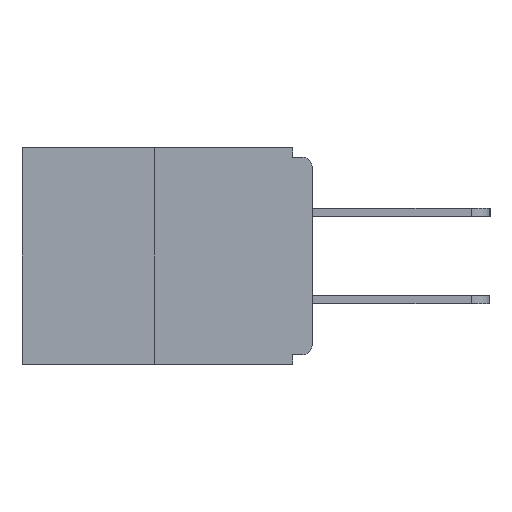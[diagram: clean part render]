
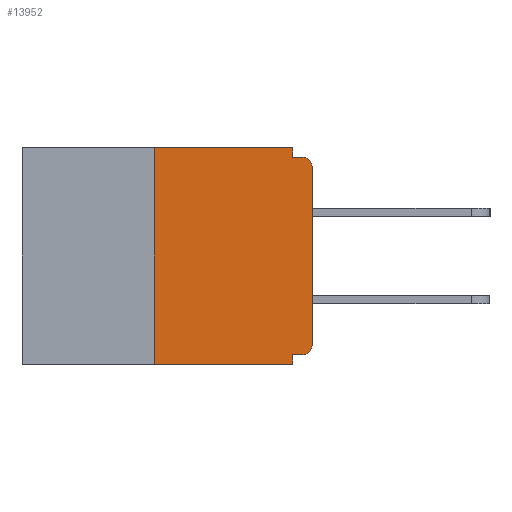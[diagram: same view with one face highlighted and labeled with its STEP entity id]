
A CAD part, left-side view. The second image highlights one B-rep face of the part: STEP entity #13952.
In plain terms, the highlighted planar face has unit normal (-1, 0, 0).
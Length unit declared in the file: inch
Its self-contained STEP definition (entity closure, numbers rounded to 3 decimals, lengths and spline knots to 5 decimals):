
#26 = CARTESIAN_POINT ( 'NONE',  ( 0., 0.46, -0.343 ) ) ;
#234 = EDGE_CURVE ( 'NONE', #9719, #2152, #12097, .T. ) ;
#257 = EDGE_CURVE ( 'NONE', #15197, #10147, #7958, .T. ) ;
#394 = CARTESIAN_POINT ( 'NONE',  ( 0., 0.25, 0. ) ) ;
#499 = DIRECTION ( 'NONE',  ( -1., 0., 0. ) ) ;
#821 = CARTESIAN_POINT ( 'NONE',  ( 0., 0.015, -0.015 ) ) ;
#1086 = CARTESIAN_POINT ( 'NONE',  ( 0., 0.25, -0.343 ) ) ;
#1186 = DIRECTION ( 'NONE',  ( 0., 0., 1. ) ) ;
#1249 = VERTEX_POINT ( 'NONE', #8671 ) ;
#1519 = CIRCLE ( 'NONE', #7314, 0.015 ) ;
#1604 = LINE ( 'NONE', #6261, #15446 ) ;
#1850 = PLANE ( 'NONE',  #8374 ) ;
#2152 = VERTEX_POINT ( 'NONE', #6568 ) ;
#2819 = VECTOR ( 'NONE', #16020, 39.37008 ) ;
#3229 = DIRECTION ( 'NONE',  ( 0., -1., 0. ) ) ;
#3533 = ORIENTED_EDGE ( 'NONE', *, *, #234, .F. ) ;
#3569 = EDGE_CURVE ( 'NONE', #5611, #10739, #1604, .T. ) ;
#3644 = VECTOR ( 'NONE', #16268, 39.37008 ) ;
#3814 = VERTEX_POINT ( 'NONE', #821 ) ;
#4016 = CARTESIAN_POINT ( 'NONE',  ( 0., 0., -0.328 ) ) ;
#4102 = ORIENTED_EDGE ( 'NONE', *, *, #6566, .T. ) ;
#4181 = EDGE_CURVE ( 'NONE', #9719, #10739, #6935, .T. ) ;
#4430 = DIRECTION ( 'NONE',  ( 0., 0., -1. ) ) ;
#4498 = LINE ( 'NONE', #4016, #2819 ) ;
#4699 = LINE ( 'NONE', #8275, #9035 ) ;
#4856 = CIRCLE ( 'NONE', #13035, 0.015 ) ;
#5150 = EDGE_CURVE ( 'NONE', #2152, #15197, #4699, .T. ) ;
#5329 = VECTOR ( 'NONE', #13283, 39.37008 ) ;
#5611 = VERTEX_POINT ( 'NONE', #9709 ) ;
#5800 = ORIENTED_EDGE ( 'NONE', *, *, #257, .F. ) ;
#6261 = CARTESIAN_POINT ( 'NONE',  ( 0., 0.031, -0.343 ) ) ;
#6269 = DIRECTION ( 'NONE',  ( 0., 0., -1. ) ) ;
#6470 = EDGE_LOOP ( 'NONE', ( #12207, #3533, #7846, #15551, #7642, #4102, #16042, #11054, #15247, #5800 ) ) ;
#6566 = EDGE_CURVE ( 'NONE', #14344, #16551, #4856, .T. ) ;
#6568 = CARTESIAN_POINT ( 'NONE',  ( 0., 0.25, 0. ) ) ;
#6770 = CARTESIAN_POINT ( 'NONE',  ( 0., 0.015, -0.328 ) ) ;
#6935 = LINE ( 'NONE', #26, #5329 ) ;
#6994 = DIRECTION ( 'NONE',  ( 0., 0., 1. ) ) ;
#7049 = CARTESIAN_POINT ( 'NONE',  ( 0., 0.031, 0. ) ) ;
#7126 = CARTESIAN_POINT ( 'NONE',  ( 0., 0.031, -0.015 ) ) ;
#7143 = DIRECTION ( 'NONE',  ( 0., 0., -1. ) ) ;
#7314 = AXIS2_PLACEMENT_3D ( 'NONE', #8338, #499, #4430 ) ;
#7642 = ORIENTED_EDGE ( 'NONE', *, *, #15091, .F. ) ;
#7813 = CARTESIAN_POINT ( 'NONE',  ( 0., 0., -0.313 ) ) ;
#7846 = ORIENTED_EDGE ( 'NONE', *, *, #4181, .T. ) ;
#7951 = FACE_OUTER_BOUND ( 'NONE', #6470, .T. ) ;
#7958 = LINE ( 'NONE', #7049, #3644 ) ;
#8275 = CARTESIAN_POINT ( 'NONE',  ( 0., 0.46, 0. ) ) ;
#8338 = CARTESIAN_POINT ( 'NONE',  ( 0., 0.015, -0.03 ) ) ;
#8374 = AXIS2_PLACEMENT_3D ( 'NONE', #12434, #15058, #7143 ) ;
#8568 = VECTOR ( 'NONE', #3229, 39.37008 ) ;
#8671 = CARTESIAN_POINT ( 'NONE',  ( 0., 0., -0.03 ) ) ;
#9035 = VECTOR ( 'NONE', #15461, 39.37008 ) ;
#9709 = CARTESIAN_POINT ( 'NONE',  ( 0., 0.031, -0.328 ) ) ;
#9719 = VERTEX_POINT ( 'NONE', #1086 ) ;
#10147 = VERTEX_POINT ( 'NONE', #7126 ) ;
#10305 = DIRECTION ( 'NONE',  ( 0., 0., -1. ) ) ;
#10739 = VERTEX_POINT ( 'NONE', #13922 ) ;
#11054 = ORIENTED_EDGE ( 'NONE', *, *, #16902, .T. ) ;
#11480 = LINE ( 'NONE', #13657, #8568 ) ;
#11542 = CARTESIAN_POINT ( 'NONE',  ( 0., 0.015, -0.313 ) ) ;
#11779 = DIRECTION ( 'NONE',  ( -1., 0., 0. ) ) ;
#11796 = EDGE_CURVE ( 'NONE', #16551, #1249, #15828, .T. ) ;
#11889 = CARTESIAN_POINT ( 'NONE',  ( 0., 0., 0. ) ) ;
#11986 = CARTESIAN_POINT ( 'NONE',  ( 0., 0.031, 0. ) ) ;
#12097 = LINE ( 'NONE', #394, #16433 ) ;
#12207 = ORIENTED_EDGE ( 'NONE', *, *, #5150, .F. ) ;
#12329 = VECTOR ( 'NONE', #1186, 39.37008 ) ;
#12434 = CARTESIAN_POINT ( 'NONE',  ( 0., 0.46, 0. ) ) ;
#13035 = AXIS2_PLACEMENT_3D ( 'NONE', #11542, #11779, #6269 ) ;
#13283 = DIRECTION ( 'NONE',  ( 0., -1., 0. ) ) ;
#13657 = CARTESIAN_POINT ( 'NONE',  ( 0., 0., -0.015 ) ) ;
#13922 = CARTESIAN_POINT ( 'NONE',  ( 0., 0.031, -0.343 ) ) ;
#13952 = ADVANCED_FACE ( 'NONE', ( #7951 ), #1850, .F. ) ;
#14344 = VERTEX_POINT ( 'NONE', #6770 ) ;
#15058 = DIRECTION ( 'NONE',  ( 1., 0., 0. ) ) ;
#15091 = EDGE_CURVE ( 'NONE', #14344, #5611, #4498, .T. ) ;
#15197 = VERTEX_POINT ( 'NONE', #11986 ) ;
#15247 = ORIENTED_EDGE ( 'NONE', *, *, #16148, .F. ) ;
#15446 = VECTOR ( 'NONE', #10305, 39.37008 ) ;
#15461 = DIRECTION ( 'NONE',  ( 0., -1., 0. ) ) ;
#15551 = ORIENTED_EDGE ( 'NONE', *, *, #3569, .F. ) ;
#15828 = LINE ( 'NONE', #11889, #12329 ) ;
#16020 = DIRECTION ( 'NONE',  ( 0., 1., 0. ) ) ;
#16042 = ORIENTED_EDGE ( 'NONE', *, *, #11796, .T. ) ;
#16148 = EDGE_CURVE ( 'NONE', #10147, #3814, #11480, .T. ) ;
#16268 = DIRECTION ( 'NONE',  ( 0., 0., -1. ) ) ;
#16433 = VECTOR ( 'NONE', #6994, 39.37008 ) ;
#16551 = VERTEX_POINT ( 'NONE', #7813 ) ;
#16902 = EDGE_CURVE ( 'NONE', #1249, #3814, #1519, .T. ) ;
